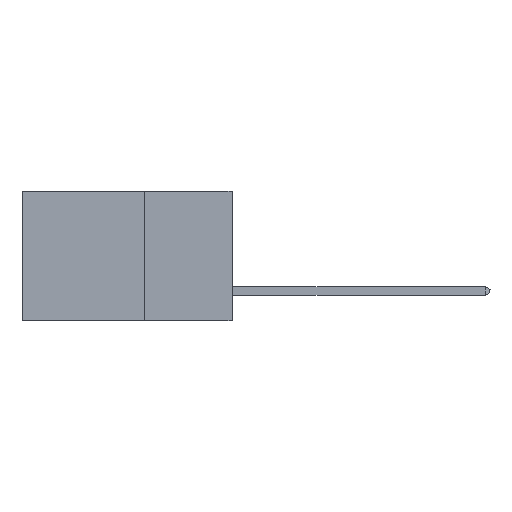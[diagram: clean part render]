
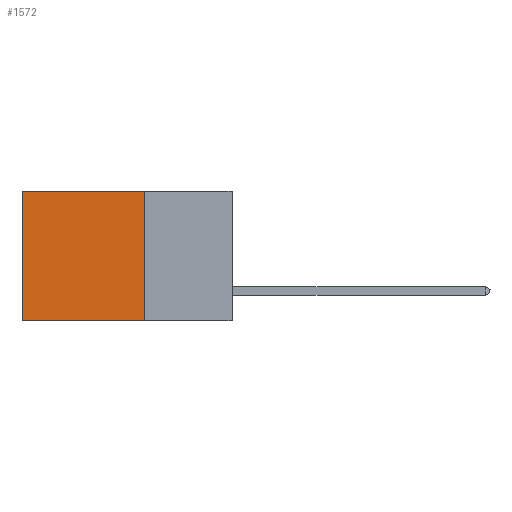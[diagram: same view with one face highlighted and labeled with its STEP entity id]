
A CAD part, left-side view. The second image highlights one B-rep face of the part: STEP entity #1572.
In plain terms, the highlighted planar face has unit normal (-1, 0, 0).
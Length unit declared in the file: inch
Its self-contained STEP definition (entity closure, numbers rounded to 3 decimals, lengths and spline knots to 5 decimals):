
#413 = EDGE_CURVE ( 'NONE', #30478, #27355, #31660, .T. ) ;
#833 = CARTESIAN_POINT ( 'NONE',  ( 0.2875, 0.25, 0. ) ) ;
#1572 = ADVANCED_FACE ( 'NONE', ( #31022 ), #35077, .F. ) ;
#1856 = ORIENTED_EDGE ( 'NONE', *, *, #40375, .F. ) ;
#2990 = CARTESIAN_POINT ( 'NONE',  ( 0.2875, 0.25, -0.37 ) ) ;
#5932 = VERTEX_POINT ( 'NONE', #10989 ) ;
#7241 = ORIENTED_EDGE ( 'NONE', *, *, #41559, .T. ) ;
#7800 = LINE ( 'NONE', #2990, #42418 ) ;
#10989 = CARTESIAN_POINT ( 'NONE',  ( 0.2875, 0.6, -0.37 ) ) ;
#11401 = CARTESIAN_POINT ( 'NONE',  ( 0.2875, 0.25, 0. ) ) ;
#11868 = DIRECTION ( 'NONE',  ( 1., 0., 0. ) ) ;
#12173 = CARTESIAN_POINT ( 'NONE',  ( 0.2875, 0.6, 0. ) ) ;
#12324 = DIRECTION ( 'NONE',  ( 0., 0., -1. ) ) ;
#12853 = VECTOR ( 'NONE', #16034, 39.37008 ) ;
#13757 = CARTESIAN_POINT ( 'NONE',  ( 0.2875, 0.6, 0. ) ) ;
#16034 = DIRECTION ( 'NONE',  ( 0., 1., 0. ) ) ;
#17085 = DIRECTION ( 'NONE',  ( 0., 0., -1. ) ) ;
#24673 = EDGE_LOOP ( 'NONE', ( #7241, #1856, #37062, #29689 ) ) ;
#25173 = CARTESIAN_POINT ( 'NONE',  ( 0.2875, 0.25, 0. ) ) ;
#27355 = VERTEX_POINT ( 'NONE', #13757 ) ;
#28122 = VECTOR ( 'NONE', #12324, 39.37008 ) ;
#28816 = AXIS2_PLACEMENT_3D ( 'NONE', #31594, #11868, #17085 ) ;
#29689 = ORIENTED_EDGE ( 'NONE', *, *, #413, .T. ) ;
#30069 = VERTEX_POINT ( 'NONE', #36482 ) ;
#30478 = VERTEX_POINT ( 'NONE', #25173 ) ;
#31022 = FACE_OUTER_BOUND ( 'NONE', #24673, .T. ) ;
#31426 = DIRECTION ( 'NONE',  ( 0., 0., -1. ) ) ;
#31594 = CARTESIAN_POINT ( 'NONE',  ( 0.2875, 0.25, 0. ) ) ;
#31660 = LINE ( 'NONE', #11401, #12853 ) ;
#32749 = LINE ( 'NONE', #833, #34820 ) ;
#33336 = EDGE_CURVE ( 'NONE', #30478, #30069, #32749, .T. ) ;
#34820 = VECTOR ( 'NONE', #31426, 39.37008 ) ;
#35077 = PLANE ( 'NONE',  #28816 ) ;
#36482 = CARTESIAN_POINT ( 'NONE',  ( 0.2875, 0.25, -0.37 ) ) ;
#37018 = LINE ( 'NONE', #12173, #28122 ) ;
#37062 = ORIENTED_EDGE ( 'NONE', *, *, #33336, .F. ) ;
#40375 = EDGE_CURVE ( 'NONE', #30069, #5932, #7800, .T. ) ;
#41559 = EDGE_CURVE ( 'NONE', #27355, #5932, #37018, .T. ) ;
#42418 = VECTOR ( 'NONE', #42938, 39.37008 ) ;
#42938 = DIRECTION ( 'NONE',  ( 0., 1., 0. ) ) ;
